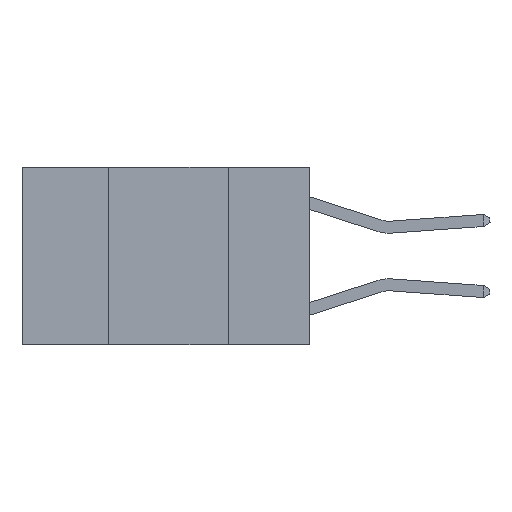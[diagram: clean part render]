
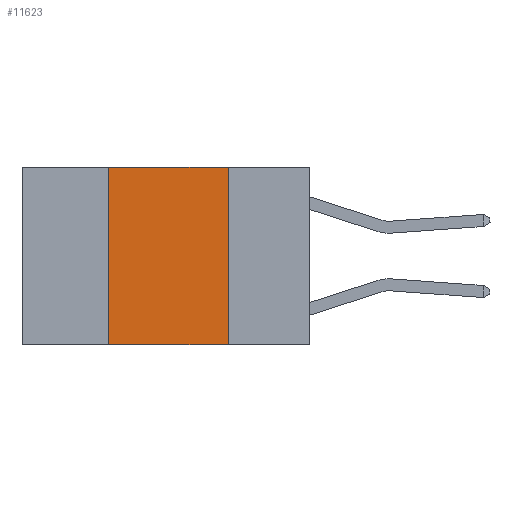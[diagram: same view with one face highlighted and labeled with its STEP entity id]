
A CAD part, left-side view. The second image highlights one B-rep face of the part: STEP entity #11623.
In plain terms, the highlighted planar face has unit normal (-1, 0, 0).
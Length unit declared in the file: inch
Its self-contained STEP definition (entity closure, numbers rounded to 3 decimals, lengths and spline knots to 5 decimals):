
#89 = EDGE_CURVE ( 'NONE', #10919, #989, #5834, .T. ) ;
#139 = DIRECTION ( 'NONE',  ( 0., -1., 0. ) ) ;
#177 = VECTOR ( 'NONE', #139, 39.37008 ) ;
#333 = DIRECTION ( 'NONE',  ( 0., 0., -1. ) ) ;
#699 = VERTEX_POINT ( 'NONE', #13248 ) ;
#848 = EDGE_CURVE ( 'NONE', #10919, #699, #3940, .T. ) ;
#989 = VERTEX_POINT ( 'NONE', #1032 ) ;
#1032 = CARTESIAN_POINT ( 'NONE',  ( 0., 0.17, -0.37 ) ) ;
#2243 = LINE ( 'NONE', #4835, #4665 ) ;
#2679 = EDGE_CURVE ( 'NONE', #699, #5975, #11124, .T. ) ;
#3025 = CARTESIAN_POINT ( 'NONE',  ( 0., 0.6, -0.37 ) ) ;
#3059 = ORIENTED_EDGE ( 'NONE', *, *, #848, .F. ) ;
#3434 = DIRECTION ( 'NONE',  ( 0., 0., 1. ) ) ;
#3703 = EDGE_CURVE ( 'NONE', #5975, #989, #2243, .T. ) ;
#3940 = LINE ( 'NONE', #10687, #11494 ) ;
#4665 = VECTOR ( 'NONE', #6844, 39.37008 ) ;
#4835 = CARTESIAN_POINT ( 'NONE',  ( 0., 0.17, 0. ) ) ;
#4872 = CARTESIAN_POINT ( 'NONE',  ( 0., 0.17, 0. ) ) ;
#5583 = ORIENTED_EDGE ( 'NONE', *, *, #89, .T. ) ;
#5834 = LINE ( 'NONE', #3025, #8576 ) ;
#5975 = VERTEX_POINT ( 'NONE', #4872 ) ;
#6482 = DIRECTION ( 'NONE',  ( 1., 0., 0. ) ) ;
#6844 = DIRECTION ( 'NONE',  ( 0., 0., -1. ) ) ;
#7930 = ORIENTED_EDGE ( 'NONE', *, *, #2679, .F. ) ;
#8521 = CARTESIAN_POINT ( 'NONE',  ( 0., 0.6, 0. ) ) ;
#8576 = VECTOR ( 'NONE', #9699, 39.37008 ) ;
#8644 = FACE_OUTER_BOUND ( 'NONE', #9789, .T. ) ;
#9699 = DIRECTION ( 'NONE',  ( 0., -1., 0. ) ) ;
#9789 = EDGE_LOOP ( 'NONE', ( #12900, #7930, #3059, #5583 ) ) ;
#10439 = CARTESIAN_POINT ( 'NONE',  ( 0., 0.6, 0. ) ) ;
#10687 = CARTESIAN_POINT ( 'NONE',  ( 0., 0.42, 0. ) ) ;
#10919 = VERTEX_POINT ( 'NONE', #12538 ) ;
#11124 = LINE ( 'NONE', #10439, #177 ) ;
#11494 = VECTOR ( 'NONE', #3434, 39.37008 ) ;
#11623 = ADVANCED_FACE ( 'NONE', ( #8644 ), #12643, .F. ) ;
#12538 = CARTESIAN_POINT ( 'NONE',  ( 0., 0.42, -0.37 ) ) ;
#12643 = PLANE ( 'NONE',  #12832 ) ;
#12832 = AXIS2_PLACEMENT_3D ( 'NONE', #8521, #6482, #333 ) ;
#12900 = ORIENTED_EDGE ( 'NONE', *, *, #3703, .F. ) ;
#13248 = CARTESIAN_POINT ( 'NONE',  ( 0., 0.42, 0. ) ) ;
